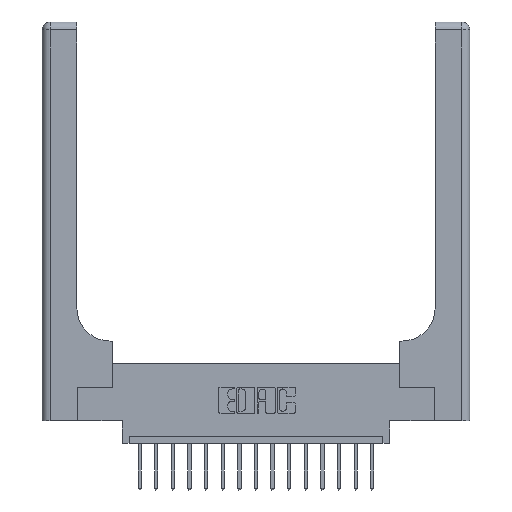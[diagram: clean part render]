
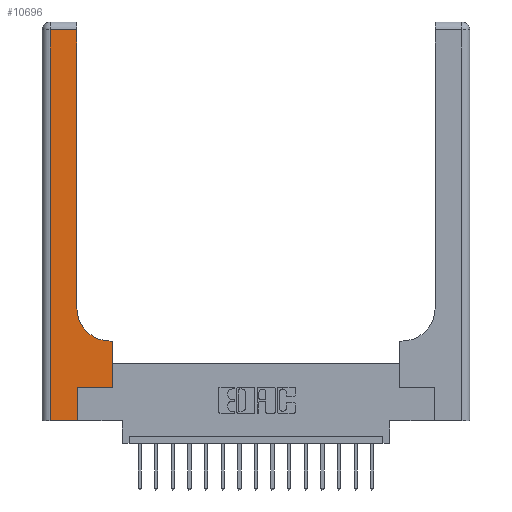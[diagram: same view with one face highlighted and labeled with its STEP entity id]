
A CAD part, top view. The second image highlights one B-rep face of the part: STEP entity #10696.
In plain terms, the highlighted planar face has unit normal (0, 0, 1).
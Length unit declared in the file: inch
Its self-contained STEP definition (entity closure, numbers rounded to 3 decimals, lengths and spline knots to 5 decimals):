
#562 = DIRECTION ( 'NONE',  ( 0., 0., -1. ) ) ;
#1047 = ORIENTED_EDGE ( 'NONE', *, *, #7682, .T. ) ;
#2193 = VERTEX_POINT ( 'NONE', #16771 ) ;
#2262 = CARTESIAN_POINT ( 'NONE',  ( 0., 3., 0.37 ) ) ;
#2452 = CARTESIAN_POINT ( 'NONE',  ( 0.06, 0., 0.37 ) ) ;
#2480 = LINE ( 'NONE', #6821, #10763 ) ;
#2665 = AXIS2_PLACEMENT_3D ( 'NONE', #2262, #562, #3597 ) ;
#2815 = EDGE_CURVE ( 'NONE', #18051, #7723, #16159, .T. ) ;
#3059 = DIRECTION ( 'NONE',  ( 1., 0., 0. ) ) ;
#3203 = ORIENTED_EDGE ( 'NONE', *, *, #7815, .T. ) ;
#3412 = DIRECTION ( 'NONE',  ( -1., 0., 0. ) ) ;
#3449 = CARTESIAN_POINT ( 'NONE',  ( 0.528, 0.6, 0.37 ) ) ;
#3500 = LINE ( 'NONE', #6234, #8073 ) ;
#3597 = DIRECTION ( 'NONE',  ( -1., 0., 0. ) ) ;
#4420 = CARTESIAN_POINT ( 'NONE',  ( 0.06, 2.94, 0.37 ) ) ;
#5618 = LINE ( 'NONE', #9682, #10027 ) ;
#5847 = VECTOR ( 'NONE', #6655, 39.37008 ) ;
#6234 = CARTESIAN_POINT ( 'NONE',  ( 0.265, 0.25, 0.37 ) ) ;
#6280 = DIRECTION ( 'NONE',  ( 0., 1., 0. ) ) ;
#6367 = ORIENTED_EDGE ( 'NONE', *, *, #2815, .T. ) ;
#6373 = VERTEX_POINT ( 'NONE', #12288 ) ;
#6655 = DIRECTION ( 'NONE',  ( 0., 1., 0. ) ) ;
#6821 = CARTESIAN_POINT ( 'NONE',  ( 0.26, 0.6, 0.37 ) ) ;
#7406 = VERTEX_POINT ( 'NONE', #3449 ) ;
#7601 = CARTESIAN_POINT ( 'NONE',  ( 0.26, 3., 0.37 ) ) ;
#7682 = EDGE_CURVE ( 'NONE', #15493, #18051, #5618, .T. ) ;
#7707 = DIRECTION ( 'NONE',  ( 0., 1., 0. ) ) ;
#7723 = VERTEX_POINT ( 'NONE', #14034 ) ;
#7815 = EDGE_CURVE ( 'NONE', #6373, #16756, #7901, .T. ) ;
#7901 = CIRCLE ( 'NONE', #8815, 0.25 ) ;
#8073 = VECTOR ( 'NONE', #14859, 39.37008 ) ;
#8657 = EDGE_CURVE ( 'NONE', #16756, #12848, #13306, .T. ) ;
#8815 = AXIS2_PLACEMENT_3D ( 'NONE', #16034, #16306, #3059 ) ;
#8901 = VECTOR ( 'NONE', #7707, 39.37008 ) ;
#9044 = CARTESIAN_POINT ( 'NONE',  ( 0.265, 0., 0.37 ) ) ;
#9076 = LINE ( 'NONE', #13439, #9897 ) ;
#9357 = ORIENTED_EDGE ( 'NONE', *, *, #15296, .T. ) ;
#9406 = DIRECTION ( 'NONE',  ( 0., -1., 0. ) ) ;
#9682 = CARTESIAN_POINT ( 'NONE',  ( 0., 0., 0.37 ) ) ;
#9764 = DIRECTION ( 'NONE',  ( -1., 0., 0. ) ) ;
#9806 = EDGE_LOOP ( 'NONE', ( #17767, #16777, #17959, #1047, #6367, #9357, #17954, #16609, #3203 ) ) ;
#9897 = VECTOR ( 'NONE', #3412, 39.37008 ) ;
#9963 = EDGE_CURVE ( 'NONE', #18408, #15493, #15367, .T. ) ;
#10027 = VECTOR ( 'NONE', #17063, 39.37008 ) ;
#10696 = ADVANCED_FACE ( 'NONE', ( #16562 ), #11058, .F. ) ;
#10763 = VECTOR ( 'NONE', #9764, 39.37008 ) ;
#11058 = PLANE ( 'NONE',  #2665 ) ;
#11293 = LINE ( 'NONE', #14131, #5847 ) ;
#12226 = EDGE_CURVE ( 'NONE', #2193, #7406, #11293, .T. ) ;
#12288 = CARTESIAN_POINT ( 'NONE',  ( 0.51, 0.6, 0.37 ) ) ;
#12848 = VERTEX_POINT ( 'NONE', #18232 ) ;
#13306 = LINE ( 'NONE', #7601, #15539 ) ;
#13439 = CARTESIAN_POINT ( 'NONE',  ( 0., 2.94, 0.37 ) ) ;
#13812 = EDGE_CURVE ( 'NONE', #7406, #6373, #2480, .T. ) ;
#14034 = CARTESIAN_POINT ( 'NONE',  ( 0.265, 0.25, 0.37 ) ) ;
#14131 = CARTESIAN_POINT ( 'NONE',  ( 0.528, 0.25, 0.37 ) ) ;
#14847 = CARTESIAN_POINT ( 'NONE',  ( 0.265, 0., 0.37 ) ) ;
#14859 = DIRECTION ( 'NONE',  ( 1., 0., 0. ) ) ;
#15218 = EDGE_CURVE ( 'NONE', #12848, #18408, #9076, .T. ) ;
#15296 = EDGE_CURVE ( 'NONE', #7723, #2193, #3500, .T. ) ;
#15367 = LINE ( 'NONE', #16879, #17681 ) ;
#15493 = VERTEX_POINT ( 'NONE', #2452 ) ;
#15539 = VECTOR ( 'NONE', #6280, 39.37008 ) ;
#16034 = CARTESIAN_POINT ( 'NONE',  ( 0.51, 0.85, 0.37 ) ) ;
#16159 = LINE ( 'NONE', #9044, #8901 ) ;
#16306 = DIRECTION ( 'NONE',  ( 0., 0., -1. ) ) ;
#16562 = FACE_OUTER_BOUND ( 'NONE', #9806, .T. ) ;
#16609 = ORIENTED_EDGE ( 'NONE', *, *, #13812, .T. ) ;
#16655 = CARTESIAN_POINT ( 'NONE',  ( 0.26, 0.85, 0.37 ) ) ;
#16756 = VERTEX_POINT ( 'NONE', #16655 ) ;
#16771 = CARTESIAN_POINT ( 'NONE',  ( 0.528, 0.25, 0.37 ) ) ;
#16777 = ORIENTED_EDGE ( 'NONE', *, *, #15218, .T. ) ;
#16879 = CARTESIAN_POINT ( 'NONE',  ( 0.06, 3., 0.37 ) ) ;
#17063 = DIRECTION ( 'NONE',  ( 1., 0., 0. ) ) ;
#17681 = VECTOR ( 'NONE', #9406, 39.37008 ) ;
#17767 = ORIENTED_EDGE ( 'NONE', *, *, #8657, .T. ) ;
#17954 = ORIENTED_EDGE ( 'NONE', *, *, #12226, .T. ) ;
#17959 = ORIENTED_EDGE ( 'NONE', *, *, #9963, .T. ) ;
#18051 = VERTEX_POINT ( 'NONE', #14847 ) ;
#18232 = CARTESIAN_POINT ( 'NONE',  ( 0.26, 2.94, 0.37 ) ) ;
#18408 = VERTEX_POINT ( 'NONE', #4420 ) ;
